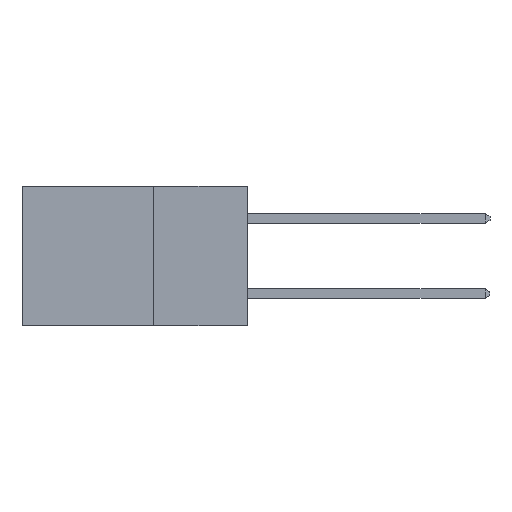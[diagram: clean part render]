
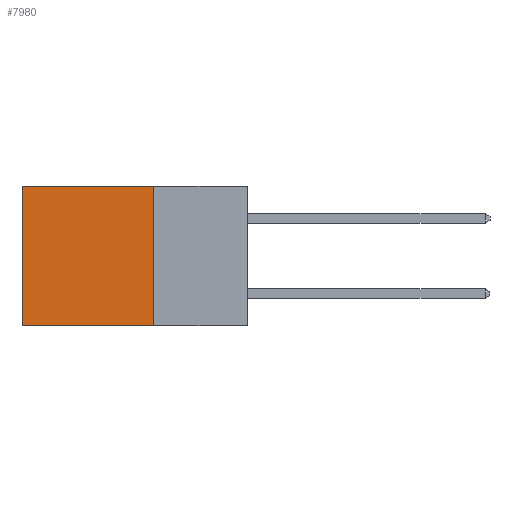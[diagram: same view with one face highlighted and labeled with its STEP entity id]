
A CAD part, left-side view. The second image highlights one B-rep face of the part: STEP entity #7980.
In plain terms, the highlighted planar face has unit normal (-1, 0, 0).
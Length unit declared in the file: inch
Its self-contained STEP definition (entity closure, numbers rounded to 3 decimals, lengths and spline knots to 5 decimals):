
#105 = FACE_OUTER_BOUND ( 'NONE', #5530, .T. ) ;
#275 = CARTESIAN_POINT ( 'NONE',  ( 0.298, 0.25, -0.37 ) ) ;
#796 = CARTESIAN_POINT ( 'NONE',  ( 0.298, 0.6, 0. ) ) ;
#1217 = EDGE_CURVE ( 'NONE', #5983, #7900, #4042, .T. ) ;
#1274 = DIRECTION ( 'NONE',  ( 0., 1., 0. ) ) ;
#1848 = VECTOR ( 'NONE', #1274, 39.37008 ) ;
#1873 = EDGE_CURVE ( 'NONE', #7900, #4373, #9811, .T. ) ;
#2889 = ORIENTED_EDGE ( 'NONE', *, *, #1217, .T. ) ;
#3486 = DIRECTION ( 'NONE',  ( 0., 0., -1. ) ) ;
#3512 = EDGE_CURVE ( 'NONE', #5983, #8383, #10410, .T. ) ;
#3766 = VECTOR ( 'NONE', #10510, 39.37008 ) ;
#4042 = LINE ( 'NONE', #9849, #3766 ) ;
#4286 = CARTESIAN_POINT ( 'NONE',  ( 0.298, 0.6, 0. ) ) ;
#4373 = VERTEX_POINT ( 'NONE', #7694 ) ;
#4592 = CARTESIAN_POINT ( 'NONE',  ( 0.298, 0.25, 0. ) ) ;
#4890 = DIRECTION ( 'NONE',  ( 0., 0., -1. ) ) ;
#5022 = VECTOR ( 'NONE', #4890, 39.37008 ) ;
#5530 = EDGE_LOOP ( 'NONE', ( #9337, #7421, #5696, #2889 ) ) ;
#5610 = AXIS2_PLACEMENT_3D ( 'NONE', #7978, #8884, #3486 ) ;
#5696 = ORIENTED_EDGE ( 'NONE', *, *, #3512, .F. ) ;
#5983 = VERTEX_POINT ( 'NONE', #10592 ) ;
#7073 = PLANE ( 'NONE',  #5610 ) ;
#7126 = EDGE_CURVE ( 'NONE', #8383, #4373, #11450, .T. ) ;
#7421 = ORIENTED_EDGE ( 'NONE', *, *, #7126, .F. ) ;
#7694 = CARTESIAN_POINT ( 'NONE',  ( 0.298, 0.6, -0.37 ) ) ;
#7900 = VERTEX_POINT ( 'NONE', #4286 ) ;
#7978 = CARTESIAN_POINT ( 'NONE',  ( 0.298, 0.25, 0. ) ) ;
#7980 = ADVANCED_FACE ( 'NONE', ( #105 ), #7073, .F. ) ;
#8070 = VECTOR ( 'NONE', #8233, 39.37008 ) ;
#8233 = DIRECTION ( 'NONE',  ( 0., 0., -1. ) ) ;
#8383 = VERTEX_POINT ( 'NONE', #11280 ) ;
#8884 = DIRECTION ( 'NONE',  ( 1., 0., 0. ) ) ;
#9337 = ORIENTED_EDGE ( 'NONE', *, *, #1873, .T. ) ;
#9811 = LINE ( 'NONE', #796, #5022 ) ;
#9849 = CARTESIAN_POINT ( 'NONE',  ( 0.298, 0.25, 0. ) ) ;
#10410 = LINE ( 'NONE', #4592, #8070 ) ;
#10510 = DIRECTION ( 'NONE',  ( 0., 1., 0. ) ) ;
#10592 = CARTESIAN_POINT ( 'NONE',  ( 0.298, 0.25, 0. ) ) ;
#11280 = CARTESIAN_POINT ( 'NONE',  ( 0.298, 0.25, -0.37 ) ) ;
#11450 = LINE ( 'NONE', #275, #1848 ) ;
